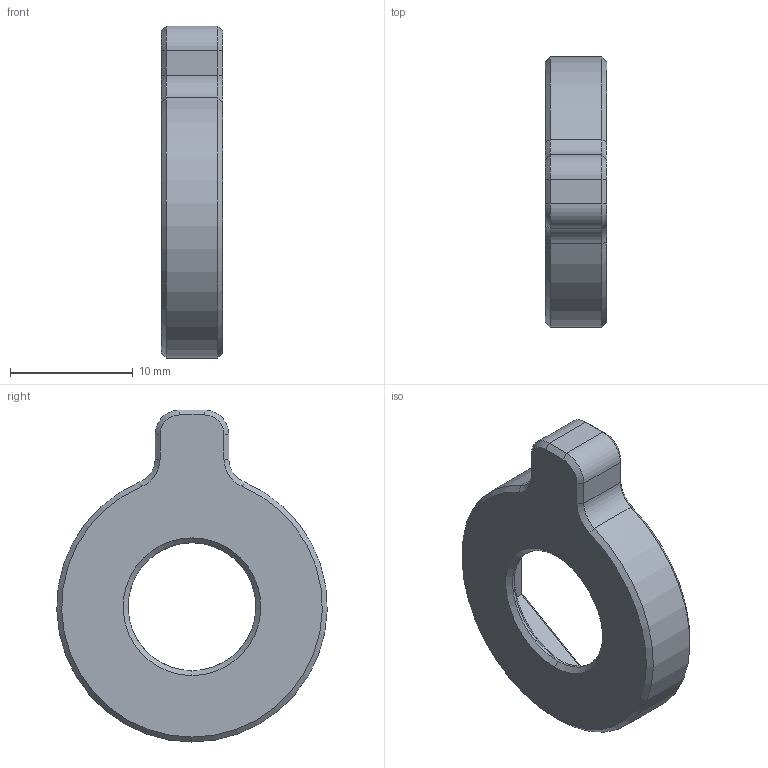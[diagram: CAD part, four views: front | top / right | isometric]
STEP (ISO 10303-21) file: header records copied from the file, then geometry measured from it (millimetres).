
FILE_DESCRIPTION(('FreeCAD Model'),'2;1');
FILE_NAME('Open CASCADE Shape Model','2022-12-07T11:23:11',('Author'),( ''),'Open CASCADE STEP processor 7.6','FreeCAD','Unknown');
FILE_SCHEMA(('AUTOMOTIVE_DESIGN { 1 0 10303 214 1 1 1 1 }'));
Length unit declared in the file: millimetre
Products named in the file (1): Barrel Selector
Bounding box: 5 x 21.99 x 27 mm (x, y, z)
Volume: 1004 mm3; surface area: 1215.1 mm2
Topology: 1 solids, 1 shells, 46 faces, 105 edges, 62 vertices
Faces by surface type: cone 16, bspline 12, plane 12, cylinder 6
Full cylindrical faces by diameter (mm): 10.4 x1
Entity records: 2583 total; most frequent: CARTESIAN_POINT 600, DIRECTION 312, ORIENTED_EDGE 210, PCURVE 210, DEFINITIONAL_REPRESENTATION 210, LINE 169, VECTOR 169, EDGE_CURVE 105
